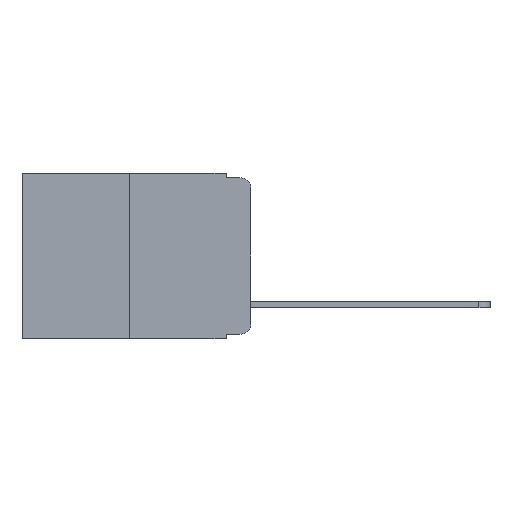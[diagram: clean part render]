
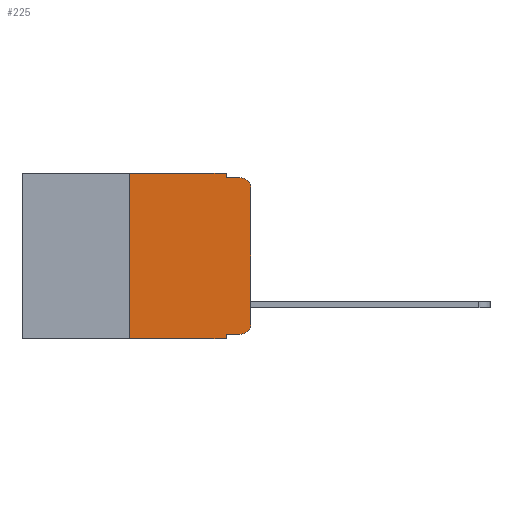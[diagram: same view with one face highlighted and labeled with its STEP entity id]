
A CAD part, left-side view. The second image highlights one B-rep face of the part: STEP entity #225.
In plain terms, the highlighted planar face has unit normal (-1, 0, 0).
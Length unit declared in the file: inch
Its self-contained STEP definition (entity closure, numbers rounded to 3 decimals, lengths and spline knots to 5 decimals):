
#135 = VERTEX_POINT ( 'NONE', #9503 ) ;
#225 = ADVANCED_FACE ( 'NONE', ( #5066 ), #12089, .F. ) ;
#1051 = EDGE_CURVE ( 'NONE', #135, #12157, #8994, .T. ) ;
#1411 = CARTESIAN_POINT ( 'NONE',  ( 0., 0.473, -0.343 ) ) ;
#1456 = LINE ( 'NONE', #10916, #11282 ) ;
#1581 = CARTESIAN_POINT ( 'NONE',  ( 0., 0.02, -0.313 ) ) ;
#1603 = VERTEX_POINT ( 'NONE', #9615 ) ;
#1665 = CARTESIAN_POINT ( 'NONE',  ( 0., 0.25, 0. ) ) ;
#1792 = DIRECTION ( 'NONE',  ( 0., -1., 0. ) ) ;
#1830 = CARTESIAN_POINT ( 'NONE',  ( 0., 0., -0.03 ) ) ;
#1922 = VECTOR ( 'NONE', #10005, 39.37008 ) ;
#2019 = EDGE_CURVE ( 'NONE', #12157, #11548, #5187, .T. ) ;
#2084 = EDGE_CURVE ( 'NONE', #3674, #1603, #5486, .T. ) ;
#2223 = LINE ( 'NONE', #1411, #1922 ) ;
#2640 = AXIS2_PLACEMENT_3D ( 'NONE', #1581, #2653, #8408 ) ;
#2653 = DIRECTION ( 'NONE',  ( -1., 0., 0. ) ) ;
#2654 = VECTOR ( 'NONE', #11301, 39.37008 ) ;
#2708 = EDGE_CURVE ( 'NONE', #4529, #6811, #1456, .T. ) ;
#2732 = VECTOR ( 'NONE', #1792, 39.37008 ) ;
#2957 = ORIENTED_EDGE ( 'NONE', *, *, #7983, .F. ) ;
#3021 = EDGE_LOOP ( 'NONE', ( #9391, #9687, #4886, #9977, #2957, #8052, #3267, #8344, #3555, #3863 ) ) ;
#3209 = CARTESIAN_POINT ( 'NONE',  ( 0., 0.473, 0. ) ) ;
#3267 = ORIENTED_EDGE ( 'NONE', *, *, #8864, .T. ) ;
#3311 = LINE ( 'NONE', #9193, #8391 ) ;
#3449 = DIRECTION ( 'NONE',  ( 0., -1., 0. ) ) ;
#3555 = ORIENTED_EDGE ( 'NONE', *, *, #8107, .T. ) ;
#3674 = VERTEX_POINT ( 'NONE', #9012 ) ;
#3863 = ORIENTED_EDGE ( 'NONE', *, *, #1051, .T. ) ;
#4082 = CARTESIAN_POINT ( 'NONE',  ( 0., 0.051, 0. ) ) ;
#4120 = DIRECTION ( 'NONE',  ( 0., 0., -1. ) ) ;
#4213 = LINE ( 'NONE', #8113, #11457 ) ;
#4416 = AXIS2_PLACEMENT_3D ( 'NONE', #9004, #7681, #4120 ) ;
#4529 = VERTEX_POINT ( 'NONE', #6426 ) ;
#4550 = DIRECTION ( 'NONE',  ( 0., 0., -1. ) ) ;
#4772 = DIRECTION ( 'NONE',  ( 0., 0., 1. ) ) ;
#4886 = ORIENTED_EDGE ( 'NONE', *, *, #11523, .F. ) ;
#5066 = FACE_OUTER_BOUND ( 'NONE', #3021, .T. ) ;
#5187 = LINE ( 'NONE', #7552, #2654 ) ;
#5284 = DIRECTION ( 'NONE',  ( -1., 0., 0. ) ) ;
#5325 = VERTEX_POINT ( 'NONE', #8956 ) ;
#5337 = CARTESIAN_POINT ( 'NONE',  ( 0., 0.051, -0.01 ) ) ;
#5486 = LINE ( 'NONE', #12186, #7146 ) ;
#5640 = CARTESIAN_POINT ( 'NONE',  ( 0., 0., -0.313 ) ) ;
#5810 = LINE ( 'NONE', #3209, #12018 ) ;
#6075 = DIRECTION ( 'NONE',  ( 0., -1., 0. ) ) ;
#6426 = CARTESIAN_POINT ( 'NONE',  ( 0., 0.25, -0.343 ) ) ;
#6811 = VERTEX_POINT ( 'NONE', #1665 ) ;
#7146 = VECTOR ( 'NONE', #4550, 39.37008 ) ;
#7552 = CARTESIAN_POINT ( 'NONE',  ( 0., 0., 0. ) ) ;
#7564 = EDGE_CURVE ( 'NONE', #10249, #8121, #4213, .T. ) ;
#7681 = DIRECTION ( 'NONE',  ( 1., 0., 0. ) ) ;
#7983 = EDGE_CURVE ( 'NONE', #6811, #10249, #5810, .T. ) ;
#8052 = ORIENTED_EDGE ( 'NONE', *, *, #2708, .F. ) ;
#8107 = EDGE_CURVE ( 'NONE', #3674, #135, #3311, .T. ) ;
#8113 = CARTESIAN_POINT ( 'NONE',  ( 0., 0.051, 0. ) ) ;
#8121 = VERTEX_POINT ( 'NONE', #5337 ) ;
#8344 = ORIENTED_EDGE ( 'NONE', *, *, #2084, .F. ) ;
#8391 = VECTOR ( 'NONE', #3449, 39.37008 ) ;
#8408 = DIRECTION ( 'NONE',  ( 0., 0., -1. ) ) ;
#8694 = EDGE_CURVE ( 'NONE', #11548, #5325, #9140, .T. ) ;
#8864 = EDGE_CURVE ( 'NONE', #4529, #1603, #2223, .T. ) ;
#8956 = CARTESIAN_POINT ( 'NONE',  ( 0., 0.02, -0.01 ) ) ;
#8994 = CIRCLE ( 'NONE', #2640, 0.02 ) ;
#9004 = CARTESIAN_POINT ( 'NONE',  ( 0., 0.473, 0. ) ) ;
#9012 = CARTESIAN_POINT ( 'NONE',  ( 0., 0.051, -0.333 ) ) ;
#9140 = CIRCLE ( 'NONE', #9545, 0.02 ) ;
#9193 = CARTESIAN_POINT ( 'NONE',  ( 0., 0.051, -0.333 ) ) ;
#9391 = ORIENTED_EDGE ( 'NONE', *, *, #2019, .T. ) ;
#9503 = CARTESIAN_POINT ( 'NONE',  ( 0., 0.02, -0.333 ) ) ;
#9545 = AXIS2_PLACEMENT_3D ( 'NONE', #10978, #5284, #11894 ) ;
#9615 = CARTESIAN_POINT ( 'NONE',  ( 0., 0.051, -0.343 ) ) ;
#9687 = ORIENTED_EDGE ( 'NONE', *, *, #8694, .T. ) ;
#9977 = ORIENTED_EDGE ( 'NONE', *, *, #7564, .F. ) ;
#10005 = DIRECTION ( 'NONE',  ( 0., -1., 0. ) ) ;
#10012 = DIRECTION ( 'NONE',  ( 0., 0., -1. ) ) ;
#10249 = VERTEX_POINT ( 'NONE', #4082 ) ;
#10654 = LINE ( 'NONE', #11271, #2732 ) ;
#10916 = CARTESIAN_POINT ( 'NONE',  ( 0., 0.25, 0. ) ) ;
#10978 = CARTESIAN_POINT ( 'NONE',  ( 0., 0.02, -0.03 ) ) ;
#11271 = CARTESIAN_POINT ( 'NONE',  ( 0., 0.051, -0.01 ) ) ;
#11282 = VECTOR ( 'NONE', #4772, 39.37008 ) ;
#11301 = DIRECTION ( 'NONE',  ( 0., 0., 1. ) ) ;
#11457 = VECTOR ( 'NONE', #10012, 39.37008 ) ;
#11523 = EDGE_CURVE ( 'NONE', #8121, #5325, #10654, .T. ) ;
#11548 = VERTEX_POINT ( 'NONE', #1830 ) ;
#11894 = DIRECTION ( 'NONE',  ( 0., 0., -1. ) ) ;
#12018 = VECTOR ( 'NONE', #6075, 39.37008 ) ;
#12089 = PLANE ( 'NONE',  #4416 ) ;
#12157 = VERTEX_POINT ( 'NONE', #5640 ) ;
#12186 = CARTESIAN_POINT ( 'NONE',  ( 0., 0.051, 0. ) ) ;
